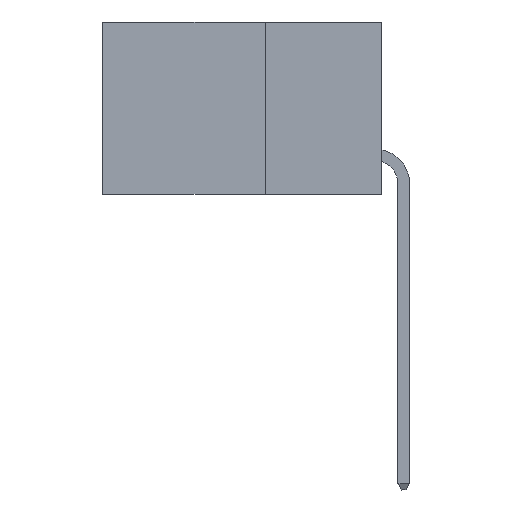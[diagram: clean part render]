
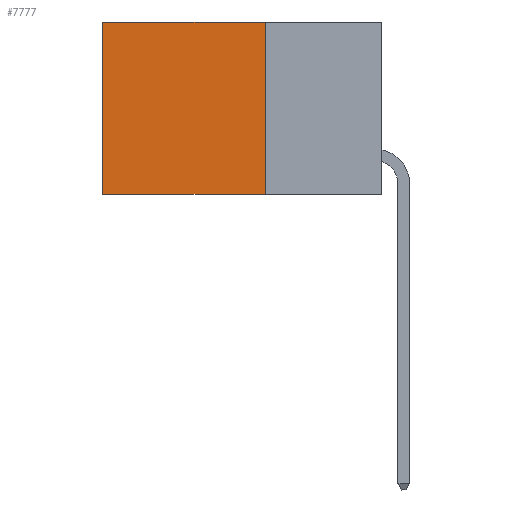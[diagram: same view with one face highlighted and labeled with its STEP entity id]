
A CAD part, left-side view. The second image highlights one B-rep face of the part: STEP entity #7777.
In plain terms, the highlighted planar face has unit normal (-1, 0, 0).
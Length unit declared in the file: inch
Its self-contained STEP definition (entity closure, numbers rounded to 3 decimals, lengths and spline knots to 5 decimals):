
#273 = VECTOR ( 'NONE', #9446, 39.37008 ) ;
#601 = LINE ( 'NONE', #8525, #273 ) ;
#2308 = ORIENTED_EDGE ( 'NONE', *, *, #10815, .F. ) ;
#2427 = PLANE ( 'NONE',  #6592 ) ;
#3191 = LINE ( 'NONE', #9979, #10514 ) ;
#3547 = EDGE_CURVE ( 'NONE', #7325, #11297, #12157, .T. ) ;
#3904 = EDGE_LOOP ( 'NONE', ( #5714, #6551, #2308, #11801 ) ) ;
#4585 = CARTESIAN_POINT ( 'NONE',  ( 0.2875, 0.25, -0.37 ) ) ;
#5182 = LINE ( 'NONE', #8930, #9956 ) ;
#5257 = EDGE_CURVE ( 'NONE', #11297, #7841, #3191, .T. ) ;
#5337 = CARTESIAN_POINT ( 'NONE',  ( 0.2875, 0.25, 0. ) ) ;
#5515 = VERTEX_POINT ( 'NONE', #4585 ) ;
#5714 = ORIENTED_EDGE ( 'NONE', *, *, #5257, .T. ) ;
#5751 = DIRECTION ( 'NONE',  ( 0., 1., 0. ) ) ;
#6337 = DIRECTION ( 'NONE',  ( 0., 0., -1. ) ) ;
#6551 = ORIENTED_EDGE ( 'NONE', *, *, #9883, .F. ) ;
#6592 = AXIS2_PLACEMENT_3D ( 'NONE', #5337, #11959, #6337 ) ;
#7325 = VERTEX_POINT ( 'NONE', #7542 ) ;
#7504 = VECTOR ( 'NONE', #5751, 39.37008 ) ;
#7542 = CARTESIAN_POINT ( 'NONE',  ( 0.2875, 0.25, 0. ) ) ;
#7777 = ADVANCED_FACE ( 'NONE', ( #11903 ), #2427, .F. ) ;
#7841 = VERTEX_POINT ( 'NONE', #12047 ) ;
#8525 = CARTESIAN_POINT ( 'NONE',  ( 0.2875, 0.25, -0.37 ) ) ;
#8930 = CARTESIAN_POINT ( 'NONE',  ( 0.2875, 0.25, 0. ) ) ;
#9446 = DIRECTION ( 'NONE',  ( 0., 1., 0. ) ) ;
#9869 = DIRECTION ( 'NONE',  ( 0., 0., -1. ) ) ;
#9883 = EDGE_CURVE ( 'NONE', #5515, #7841, #601, .T. ) ;
#9956 = VECTOR ( 'NONE', #9869, 39.37008 ) ;
#9979 = CARTESIAN_POINT ( 'NONE',  ( 0.2875, 0.6, 0. ) ) ;
#10514 = VECTOR ( 'NONE', #10904, 39.37008 ) ;
#10815 = EDGE_CURVE ( 'NONE', #7325, #5515, #5182, .T. ) ;
#10904 = DIRECTION ( 'NONE',  ( 0., 0., -1. ) ) ;
#11297 = VERTEX_POINT ( 'NONE', #12279 ) ;
#11801 = ORIENTED_EDGE ( 'NONE', *, *, #3547, .T. ) ;
#11903 = FACE_OUTER_BOUND ( 'NONE', #3904, .T. ) ;
#11959 = DIRECTION ( 'NONE',  ( 1., 0., 0. ) ) ;
#12047 = CARTESIAN_POINT ( 'NONE',  ( 0.2875, 0.6, -0.37 ) ) ;
#12157 = LINE ( 'NONE', #12354, #7504 ) ;
#12279 = CARTESIAN_POINT ( 'NONE',  ( 0.2875, 0.6, 0. ) ) ;
#12354 = CARTESIAN_POINT ( 'NONE',  ( 0.2875, 0.25, 0. ) ) ;
